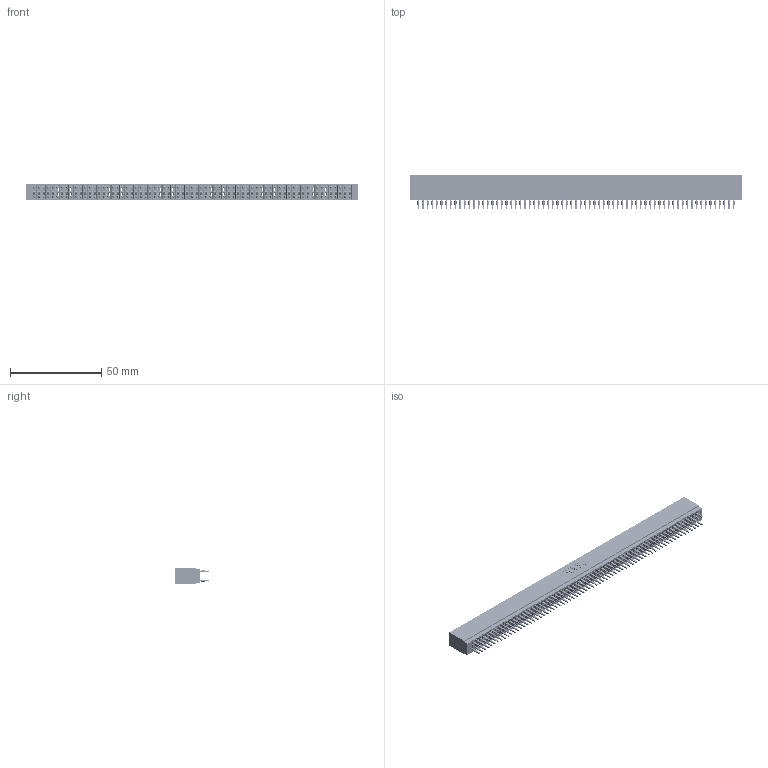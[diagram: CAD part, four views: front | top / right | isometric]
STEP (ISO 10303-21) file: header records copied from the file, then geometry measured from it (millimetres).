
FILE_DESCRIPTION (( 'STEP AP203' ), '1' );
FILE_NAME ('725-138-560-201.STEP', '2026-02-25T21:39:58', ( '' ), ( '' ), 'SwSTEP 2.0', 'SolidWorks 2023', '' );
FILE_SCHEMA (( 'CONFIG_CONTROL_DESIGN' ));
Products named in the file (3): 725-138-560-201; 745-292-001_560; 725 Part_Insulator Option - 01
Assembly tree (139 placements, depth 2):
  725-138-560-201
    725 Part_Insulator Option - 01
    745-292-001_560  x138
Bounding box: 181.86 x 18.8 x 8.89 mm (x, y, z)
Volume: 14795.8 mm3; surface area: 34003.9 mm2
Topology: 139 solids, 139 shells, 13688 faces, 37445 edges, 23766 vertices
Faces by surface type: plane 7093, cylinder 3007, bspline 2760, torus 828
Entity records: 112764 total; most frequent: CARTESIAN_POINT 20053, ORIENTED_EDGE 19542, DIRECTION 17055, EDGE_CURVE 9771, VECTOR 9167, LINE 9167, VERTEX_POINT 6230, AXIS2_PLACEMENT_3D 3944
